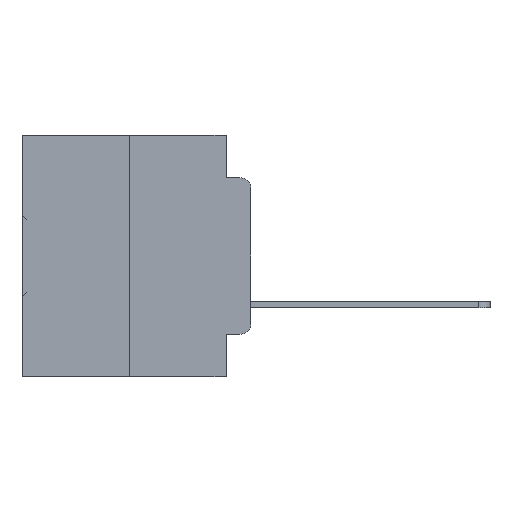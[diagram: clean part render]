
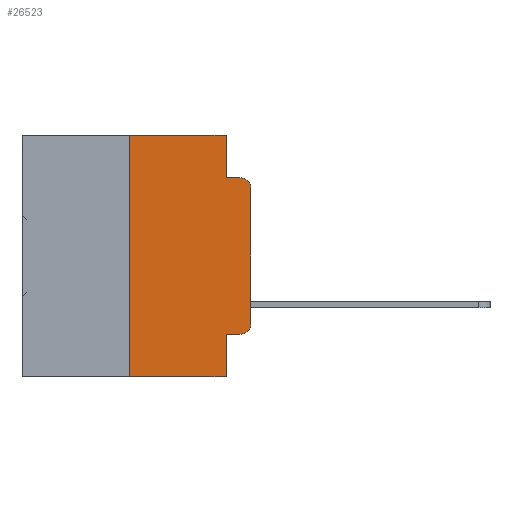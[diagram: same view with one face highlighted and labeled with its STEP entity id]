
A CAD part, left-side view. The second image highlights one B-rep face of the part: STEP entity #26523.
In plain terms, the highlighted planar face has unit normal (-1, 0, 0).
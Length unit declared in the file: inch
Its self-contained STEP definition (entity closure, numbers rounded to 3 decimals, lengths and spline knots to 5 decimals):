
#637 = VECTOR ( 'NONE', #2418, 39.37008 ) ;
#1630 = CARTESIAN_POINT ( 'NONE',  ( 0., 0.02, -0.3915 ) ) ;
#1865 = CIRCLE ( 'NONE', #20136, 0.02 ) ;
#2082 = ORIENTED_EDGE ( 'NONE', *, *, #27294, .F. ) ;
#2195 = CARTESIAN_POINT ( 'NONE',  ( 0., 0.051, -0.0885 ) ) ;
#2344 = DIRECTION ( 'NONE',  ( 0., 0., -1. ) ) ;
#2418 = DIRECTION ( 'NONE',  ( 0., -1., 0. ) ) ;
#3640 = PLANE ( 'NONE',  #29061 ) ;
#4021 = VECTOR ( 'NONE', #28416, 39.37008 ) ;
#4806 = ORIENTED_EDGE ( 'NONE', *, *, #8355, .F. ) ;
#5299 = ORIENTED_EDGE ( 'NONE', *, *, #32878, .T. ) ;
#5417 = EDGE_CURVE ( 'NONE', #20196, #18245, #13873, .T. ) ;
#5508 = CARTESIAN_POINT ( 'NONE',  ( 0., 0.051, -0.0885 ) ) ;
#6325 = VECTOR ( 'NONE', #26140, 39.37008 ) ;
#6518 = EDGE_CURVE ( 'NONE', #17930, #27701, #1865, .T. ) ;
#6560 = DIRECTION ( 'NONE',  ( 1., 0., 0. ) ) ;
#6601 = VERTEX_POINT ( 'NONE', #2195 ) ;
#6611 = ORIENTED_EDGE ( 'NONE', *, *, #17275, .F. ) ;
#6735 = CARTESIAN_POINT ( 'NONE',  ( 0., 0.051, -0.4115 ) ) ;
#6818 = DIRECTION ( 'NONE',  ( 0., 0., -1. ) ) ;
#7562 = DIRECTION ( 'NONE',  ( 0., 0., -1. ) ) ;
#8355 = EDGE_CURVE ( 'NONE', #23752, #6601, #31867, .T. ) ;
#9025 = LINE ( 'NONE', #33428, #4021 ) ;
#10032 = CARTESIAN_POINT ( 'NONE',  ( 0., 0.02, -0.4115 ) ) ;
#11613 = CARTESIAN_POINT ( 'NONE',  ( 0., 0.051, 0. ) ) ;
#11710 = VERTEX_POINT ( 'NONE', #30087 ) ;
#11987 = DIRECTION ( 'NONE',  ( 0., 0., 1. ) ) ;
#12178 = CARTESIAN_POINT ( 'NONE',  ( 0., 0.051, 0. ) ) ;
#12801 = LINE ( 'NONE', #6735, #30143 ) ;
#12896 = VERTEX_POINT ( 'NONE', #16714 ) ;
#13030 = EDGE_CURVE ( 'NONE', #18245, #17930, #22826, .T. ) ;
#13873 = CIRCLE ( 'NONE', #27356, 0.02 ) ;
#14154 = EDGE_CURVE ( 'NONE', #6601, #27701, #30810, .T. ) ;
#15578 = CARTESIAN_POINT ( 'NONE',  ( 0., 0.051, -0.5 ) ) ;
#16714 = CARTESIAN_POINT ( 'NONE',  ( 0., 0.25, -0.5 ) ) ;
#17275 = EDGE_CURVE ( 'NONE', #12896, #21692, #9025, .T. ) ;
#17301 = CARTESIAN_POINT ( 'NONE',  ( 0., 0.051, 0. ) ) ;
#17844 = VECTOR ( 'NONE', #11987, 39.37008 ) ;
#17930 = VERTEX_POINT ( 'NONE', #19187 ) ;
#18245 = VERTEX_POINT ( 'NONE', #18900 ) ;
#18609 = VECTOR ( 'NONE', #2344, 39.37008 ) ;
#18900 = CARTESIAN_POINT ( 'NONE',  ( 0., 0., -0.3915 ) ) ;
#18927 = ORIENTED_EDGE ( 'NONE', *, *, #13030, .T. ) ;
#19187 = CARTESIAN_POINT ( 'NONE',  ( 0., 0., -0.1085 ) ) ;
#19210 = DIRECTION ( 'NONE',  ( 0., -1., 0. ) ) ;
#19395 = DIRECTION ( 'NONE',  ( -1., 0., 0. ) ) ;
#19452 = VERTEX_POINT ( 'NONE', #15578 ) ;
#20136 = AXIS2_PLACEMENT_3D ( 'NONE', #28497, #25565, #7562 ) ;
#20196 = VERTEX_POINT ( 'NONE', #10032 ) ;
#21692 = VERTEX_POINT ( 'NONE', #22740 ) ;
#22482 = ORIENTED_EDGE ( 'NONE', *, *, #33501, .F. ) ;
#22527 = DIRECTION ( 'NONE',  ( 0., -1., 0. ) ) ;
#22740 = CARTESIAN_POINT ( 'NONE',  ( 0., 0.25, 0. ) ) ;
#22826 = LINE ( 'NONE', #29457, #17844 ) ;
#23325 = EDGE_CURVE ( 'NONE', #12896, #19452, #23439, .T. ) ;
#23439 = LINE ( 'NONE', #30846, #30295 ) ;
#23752 = VERTEX_POINT ( 'NONE', #12178 ) ;
#24306 = CARTESIAN_POINT ( 'NONE',  ( 0., 0.473, 0. ) ) ;
#24831 = EDGE_LOOP ( 'NONE', ( #18927, #32394, #35068, #4806, #2082, #6611, #28169, #22482, #5299, #25797 ) ) ;
#25565 = DIRECTION ( 'NONE',  ( -1., 0., 0. ) ) ;
#25797 = ORIENTED_EDGE ( 'NONE', *, *, #5417, .T. ) ;
#26140 = DIRECTION ( 'NONE',  ( 0., 0., -1. ) ) ;
#26363 = LINE ( 'NONE', #36993, #27295 ) ;
#26523 = ADVANCED_FACE ( 'NONE', ( #33326 ), #3640, .F. ) ;
#27294 = EDGE_CURVE ( 'NONE', #21692, #23752, #26363, .T. ) ;
#27295 = VECTOR ( 'NONE', #22527, 39.37008 ) ;
#27356 = AXIS2_PLACEMENT_3D ( 'NONE', #1630, #19395, #30654 ) ;
#27701 = VERTEX_POINT ( 'NONE', #30606 ) ;
#28169 = ORIENTED_EDGE ( 'NONE', *, *, #23325, .T. ) ;
#28416 = DIRECTION ( 'NONE',  ( 0., 0., 1. ) ) ;
#28497 = CARTESIAN_POINT ( 'NONE',  ( 0., 0.02, -0.1085 ) ) ;
#29061 = AXIS2_PLACEMENT_3D ( 'NONE', #24306, #6560, #6818 ) ;
#29457 = CARTESIAN_POINT ( 'NONE',  ( 0., 0., 0. ) ) ;
#30087 = CARTESIAN_POINT ( 'NONE',  ( 0., 0.051, -0.4115 ) ) ;
#30143 = VECTOR ( 'NONE', #33436, 39.37008 ) ;
#30295 = VECTOR ( 'NONE', #19210, 39.37008 ) ;
#30606 = CARTESIAN_POINT ( 'NONE',  ( 0., 0.02, -0.0885 ) ) ;
#30654 = DIRECTION ( 'NONE',  ( 0., 0., -1. ) ) ;
#30810 = LINE ( 'NONE', #5508, #637 ) ;
#30846 = CARTESIAN_POINT ( 'NONE',  ( 0., 0.473, -0.5 ) ) ;
#31867 = LINE ( 'NONE', #17301, #18609 ) ;
#32394 = ORIENTED_EDGE ( 'NONE', *, *, #6518, .T. ) ;
#32878 = EDGE_CURVE ( 'NONE', #11710, #20196, #12801, .T. ) ;
#33326 = FACE_OUTER_BOUND ( 'NONE', #24831, .T. ) ;
#33428 = CARTESIAN_POINT ( 'NONE',  ( 0., 0.25, 0. ) ) ;
#33436 = DIRECTION ( 'NONE',  ( 0., -1., 0. ) ) ;
#33501 = EDGE_CURVE ( 'NONE', #11710, #19452, #34229, .T. ) ;
#34229 = LINE ( 'NONE', #11613, #6325 ) ;
#35068 = ORIENTED_EDGE ( 'NONE', *, *, #14154, .F. ) ;
#36993 = CARTESIAN_POINT ( 'NONE',  ( 0., 0.473, 0. ) ) ;
